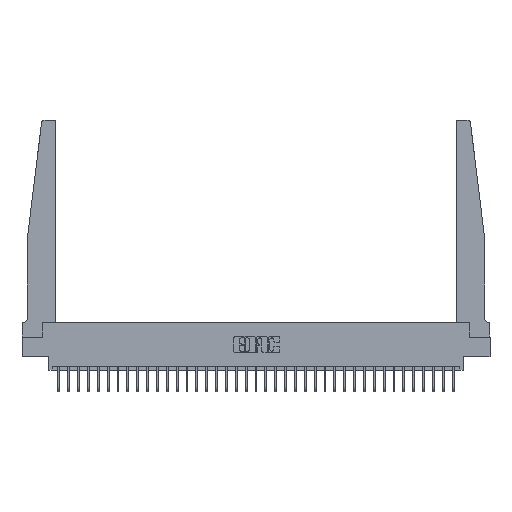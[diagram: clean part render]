
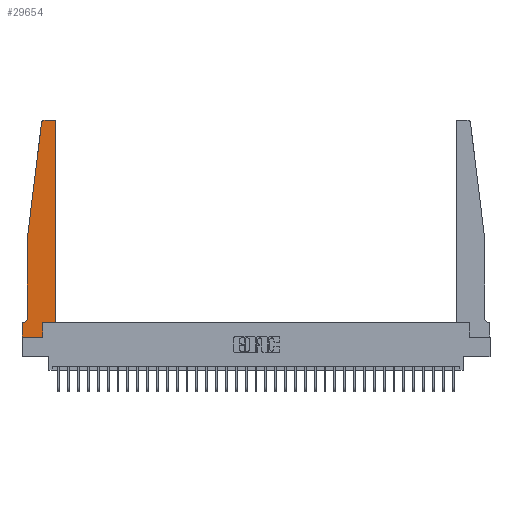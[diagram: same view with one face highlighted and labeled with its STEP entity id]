
A CAD part, top view. The second image highlights one B-rep face of the part: STEP entity #29654.
In plain terms, the highlighted planar face has unit normal (0, 0, 1).
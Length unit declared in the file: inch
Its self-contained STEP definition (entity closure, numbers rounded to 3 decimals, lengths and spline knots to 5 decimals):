
#198 = CARTESIAN_POINT ( 'NONE',  ( 0.065, 1.25, 0.37 ) ) ;
#659 = EDGE_CURVE ( 'NONE', #16058, #22111, #25555, .T. ) ;
#1365 = VECTOR ( 'NONE', #24126, 39.37008 ) ;
#1699 = CIRCLE ( 'NONE', #27265, 0.03 ) ;
#1843 = ORIENTED_EDGE ( 'NONE', *, *, #21802, .T. ) ;
#2267 = VECTOR ( 'NONE', #29332, 39.37008 ) ;
#2408 = CARTESIAN_POINT ( 'NONE',  ( 0.395, 2.75, 0.37 ) ) ;
#2640 = CARTESIAN_POINT ( 'NONE',  ( 0.425, 0.18, 0.37 ) ) ;
#3037 = CARTESIAN_POINT ( 'NONE',  ( 0.065, 0.2375, 0.37 ) ) ;
#3131 = CARTESIAN_POINT ( 'NONE',  ( 0., 0.1875, 0.37 ) ) ;
#3309 = ORIENTED_EDGE ( 'NONE', *, *, #7818, .T. ) ;
#3877 = LINE ( 'NONE', #24900, #14901 ) ;
#4350 = CARTESIAN_POINT ( 'NONE',  ( 0.27653, 2.72, 0.37 ) ) ;
#4428 = ORIENTED_EDGE ( 'NONE', *, *, #28718, .T. ) ;
#5286 = CARTESIAN_POINT ( 'NONE',  ( 0.015, 0.2375, 0.37 ) ) ;
#5295 = CARTESIAN_POINT ( 'NONE',  ( 0.065, 1.25, 0.37 ) ) ;
#5532 = DIRECTION ( 'NONE',  ( 1., 0., 0. ) ) ;
#5659 = LINE ( 'NONE', #8162, #25185 ) ;
#6175 = DIRECTION ( 'NONE',  ( 0., 1., 0. ) ) ;
#6643 = ORIENTED_EDGE ( 'NONE', *, *, #16869, .T. ) ;
#6710 = DIRECTION ( 'NONE',  ( 1., 0., 0. ) ) ;
#6828 = EDGE_CURVE ( 'NONE', #23469, #23101, #8549, .T. ) ;
#7131 = VECTOR ( 'NONE', #19061, 39.37008 ) ;
#7657 = DIRECTION ( 'NONE',  ( -1., 0., 0. ) ) ;
#7818 = EDGE_CURVE ( 'NONE', #10616, #20696, #22625, .T. ) ;
#8011 = EDGE_CURVE ( 'NONE', #23075, #10616, #5659, .T. ) ;
#8162 = CARTESIAN_POINT ( 'NONE',  ( 0., 0., 0.37 ) ) ;
#8549 = LINE ( 'NONE', #17561, #2267 ) ;
#9074 = DIRECTION ( 'NONE',  ( 0., 0., 1. ) ) ;
#10159 = EDGE_CURVE ( 'NONE', #22793, #16058, #30580, .T. ) ;
#10251 = DIRECTION ( 'NONE',  ( 0., 1., 0. ) ) ;
#10503 = EDGE_LOOP ( 'NONE', ( #28754, #4428, #6643, #13612, #19916, #1843, #21397, #3309, #15829, #22884, #29131, #18785 ) ) ;
#10616 = VERTEX_POINT ( 'NONE', #15882 ) ;
#12622 = LINE ( 'NONE', #198, #7131 ) ;
#12874 = CARTESIAN_POINT ( 'NONE',  ( 0.065, 0.1875, 0.37 ) ) ;
#12917 = VERTEX_POINT ( 'NONE', #28581 ) ;
#12996 = VECTOR ( 'NONE', #10251, 39.37008 ) ;
#13612 = ORIENTED_EDGE ( 'NONE', *, *, #19459, .T. ) ;
#14342 = VERTEX_POINT ( 'NONE', #3037 ) ;
#14901 = VECTOR ( 'NONE', #6175, 39.37008 ) ;
#14924 = AXIS2_PLACEMENT_3D ( 'NONE', #23199, #9074, #25558 ) ;
#14964 = CARTESIAN_POINT ( 'NONE',  ( 0.27653, 2.75, 0.37 ) ) ;
#15812 = LINE ( 'NONE', #12874, #24684 ) ;
#15829 = ORIENTED_EDGE ( 'NONE', *, *, #24372, .T. ) ;
#15882 = CARTESIAN_POINT ( 'NONE',  ( 0., 0., 0.37 ) ) ;
#16058 = VERTEX_POINT ( 'NONE', #2640 ) ;
#16379 = CARTESIAN_POINT ( 'NONE',  ( 0., 0., 0.37 ) ) ;
#16448 = DIRECTION ( 'NONE',  ( 1., 0., 0. ) ) ;
#16869 = EDGE_CURVE ( 'NONE', #28292, #29375, #20185, .T. ) ;
#17122 = CARTESIAN_POINT ( 'NONE',  ( 0.2605, 0., 0.37 ) ) ;
#17328 = CARTESIAN_POINT ( 'NONE',  ( 0.425, 0.18, 0.37 ) ) ;
#17561 = CARTESIAN_POINT ( 'NONE',  ( 0.25, 2.75, 0.37 ) ) ;
#18623 = CARTESIAN_POINT ( 'NONE',  ( 0.425, 2.72, 0.37 ) ) ;
#18753 = VECTOR ( 'NONE', #16448, 39.37008 ) ;
#18785 = ORIENTED_EDGE ( 'NONE', *, *, #23973, .T. ) ;
#19061 = DIRECTION ( 'NONE',  ( 0., -1., 0. ) ) ;
#19459 = EDGE_CURVE ( 'NONE', #29375, #14342, #12622, .T. ) ;
#19627 = DIRECTION ( 'NONE',  ( 0., 0., 1. ) ) ;
#19707 = FACE_OUTER_BOUND ( 'NONE', #10503, .T. ) ;
#19916 = ORIENTED_EDGE ( 'NONE', *, *, #25545, .T. ) ;
#20185 = LINE ( 'NONE', #5295, #1365 ) ;
#20696 = VERTEX_POINT ( 'NONE', #17122 ) ;
#20815 = DIRECTION ( 'NONE',  ( 0., 0., 1. ) ) ;
#21058 = CARTESIAN_POINT ( 'NONE',  ( 0.24675, 2.72367, 0.37 ) ) ;
#21140 = DIRECTION ( 'NONE',  ( 1., 0., 0. ) ) ;
#21397 = ORIENTED_EDGE ( 'NONE', *, *, #8011, .T. ) ;
#21745 = DIRECTION ( 'NONE',  ( 0., 0., -1. ) ) ;
#21802 = EDGE_CURVE ( 'NONE', #12917, #23075, #15812, .T. ) ;
#21910 = CIRCLE ( 'NONE', #25235, 0.05 ) ;
#22111 = VERTEX_POINT ( 'NONE', #18623 ) ;
#22264 = DIRECTION ( 'NONE',  ( 0., -1., 0. ) ) ;
#22625 = LINE ( 'NONE', #16379, #23370 ) ;
#22793 = VERTEX_POINT ( 'NONE', #23364 ) ;
#22884 = ORIENTED_EDGE ( 'NONE', *, *, #10159, .T. ) ;
#23075 = VERTEX_POINT ( 'NONE', #26628 ) ;
#23101 = VERTEX_POINT ( 'NONE', #14964 ) ;
#23199 = CARTESIAN_POINT ( 'NONE',  ( 0.395, 2.72, 0.37 ) ) ;
#23364 = CARTESIAN_POINT ( 'NONE',  ( 0.2605, 0.18, 0.37 ) ) ;
#23365 = CARTESIAN_POINT ( 'NONE',  ( 0.065, 1.25, 0.37 ) ) ;
#23370 = VECTOR ( 'NONE', #21140, 39.37008 ) ;
#23469 = VERTEX_POINT ( 'NONE', #2408 ) ;
#23973 = EDGE_CURVE ( 'NONE', #22111, #23469, #26746, .T. ) ;
#24126 = DIRECTION ( 'NONE',  ( -0.122, -0.992, 0. ) ) ;
#24372 = EDGE_CURVE ( 'NONE', #20696, #22793, #3877, .T. ) ;
#24684 = VECTOR ( 'NONE', #29388, 39.37008 ) ;
#24900 = CARTESIAN_POINT ( 'NONE',  ( 0.2605, 0.18, 0.37 ) ) ;
#25185 = VECTOR ( 'NONE', #22264, 39.37008 ) ;
#25235 = AXIS2_PLACEMENT_3D ( 'NONE', #5286, #21745, #7657 ) ;
#25545 = EDGE_CURVE ( 'NONE', #14342, #12917, #21910, .T. ) ;
#25555 = LINE ( 'NONE', #17328, #12996 ) ;
#25558 = DIRECTION ( 'NONE',  ( 1., 0., 0. ) ) ;
#26628 = CARTESIAN_POINT ( 'NONE',  ( 0., 0.1875, 0.37 ) ) ;
#26746 = CIRCLE ( 'NONE', #14924, 0.03 ) ;
#27090 = AXIS2_PLACEMENT_3D ( 'NONE', #3131, #19627, #5532 ) ;
#27265 = AXIS2_PLACEMENT_3D ( 'NONE', #4350, #20815, #6710 ) ;
#28292 = VERTEX_POINT ( 'NONE', #21058 ) ;
#28581 = CARTESIAN_POINT ( 'NONE',  ( 0.015, 0.1875, 0.37 ) ) ;
#28718 = EDGE_CURVE ( 'NONE', #23101, #28292, #1699, .T. ) ;
#28754 = ORIENTED_EDGE ( 'NONE', *, *, #6828, .T. ) ;
#29001 = PLANE ( 'NONE',  #27090 ) ;
#29131 = ORIENTED_EDGE ( 'NONE', *, *, #659, .T. ) ;
#29332 = DIRECTION ( 'NONE',  ( -1., 0., 0. ) ) ;
#29375 = VERTEX_POINT ( 'NONE', #23365 ) ;
#29388 = DIRECTION ( 'NONE',  ( -1., 0., 0. ) ) ;
#29654 = ADVANCED_FACE ( 'NONE', ( #19707 ), #29001, .T. ) ;
#30580 = LINE ( 'NONE', #30581, #18753 ) ;
#30581 = CARTESIAN_POINT ( 'NONE',  ( 0.425, 0.18, 0.37 ) ) ;
